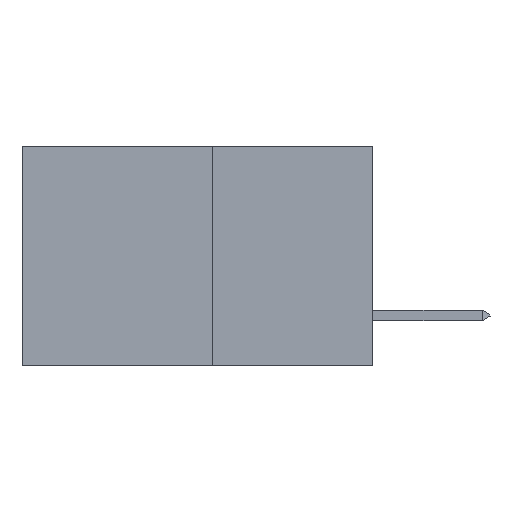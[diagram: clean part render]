
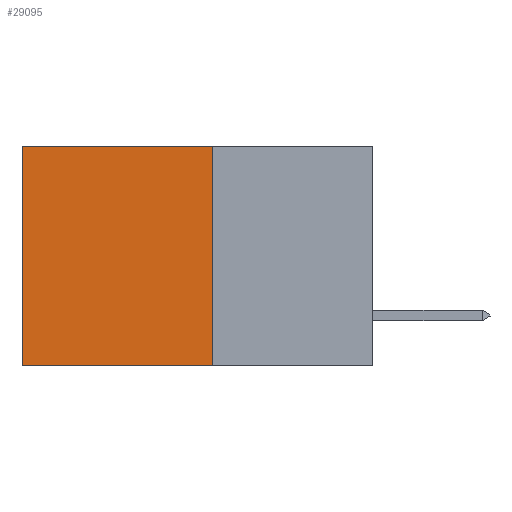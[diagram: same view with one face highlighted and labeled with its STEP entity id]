
A CAD part, left-side view. The second image highlights one B-rep face of the part: STEP entity #29095.
In plain terms, the highlighted planar face has unit normal (-1, 0, 0).
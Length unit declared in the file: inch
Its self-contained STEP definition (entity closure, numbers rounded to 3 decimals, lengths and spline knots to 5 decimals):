
#721 = ORIENTED_EDGE ( 'NONE', *, *, #19564, .F. ) ;
#1201 = VECTOR ( 'NONE', #18726, 39.37008 ) ;
#2480 = DIRECTION ( 'NONE',  ( 0., 0., -1. ) ) ;
#2927 = LINE ( 'NONE', #10168, #8708 ) ;
#3611 = VERTEX_POINT ( 'NONE', #15338 ) ;
#4893 = CARTESIAN_POINT ( 'NONE',  ( 0.277, 0.59, 0. ) ) ;
#6789 = EDGE_CURVE ( 'NONE', #23479, #3611, #12079, .T. ) ;
#7632 = CARTESIAN_POINT ( 'NONE',  ( 0.277, 0.27, -0.37 ) ) ;
#7766 = LINE ( 'NONE', #23638, #1201 ) ;
#7844 = CARTESIAN_POINT ( 'NONE',  ( 0.277, 0.59, -0.37 ) ) ;
#7878 = ORIENTED_EDGE ( 'NONE', *, *, #25058, .T. ) ;
#8621 = CARTESIAN_POINT ( 'NONE',  ( 0.277, 0.27, -0.37 ) ) ;
#8708 = VECTOR ( 'NONE', #20079, 39.37008 ) ;
#9586 = VECTOR ( 'NONE', #2480, 39.37008 ) ;
#10168 = CARTESIAN_POINT ( 'NONE',  ( 0.277, 0.27, -0.37 ) ) ;
#11098 = ORIENTED_EDGE ( 'NONE', *, *, #6789, .F. ) ;
#12079 = LINE ( 'NONE', #8621, #17922 ) ;
#12637 = DIRECTION ( 'NONE',  ( 1., 0., 0. ) ) ;
#13516 = DIRECTION ( 'NONE',  ( 0., 1., 0. ) ) ;
#15338 = CARTESIAN_POINT ( 'NONE',  ( 0.277, 0.59, -0.37 ) ) ;
#17259 = EDGE_LOOP ( 'NONE', ( #18206, #11098, #721, #7878 ) ) ;
#17922 = VECTOR ( 'NONE', #13516, 39.37008 ) ;
#18206 = ORIENTED_EDGE ( 'NONE', *, *, #26479, .T. ) ;
#18726 = DIRECTION ( 'NONE',  ( 0., 1., 0. ) ) ;
#19495 = VERTEX_POINT ( 'NONE', #4893 ) ;
#19564 = EDGE_CURVE ( 'NONE', #30369, #23479, #2927, .T. ) ;
#20079 = DIRECTION ( 'NONE',  ( 0., 0., -1. ) ) ;
#20743 = FACE_OUTER_BOUND ( 'NONE', #17259, .T. ) ;
#20803 = AXIS2_PLACEMENT_3D ( 'NONE', #7632, #12637, #29971 ) ;
#22065 = CARTESIAN_POINT ( 'NONE',  ( 0.277, 0.27, -0.37 ) ) ;
#23479 = VERTEX_POINT ( 'NONE', #22065 ) ;
#23638 = CARTESIAN_POINT ( 'NONE',  ( 0.277, 0.27, 0. ) ) ;
#25058 = EDGE_CURVE ( 'NONE', #30369, #19495, #7766, .T. ) ;
#26424 = CARTESIAN_POINT ( 'NONE',  ( 0.277, 0.27, 0. ) ) ;
#26479 = EDGE_CURVE ( 'NONE', #19495, #3611, #29401, .T. ) ;
#27534 = PLANE ( 'NONE',  #20803 ) ;
#29095 = ADVANCED_FACE ( 'NONE', ( #20743 ), #27534, .F. ) ;
#29401 = LINE ( 'NONE', #7844, #9586 ) ;
#29971 = DIRECTION ( 'NONE',  ( 0., 0., -1. ) ) ;
#30369 = VERTEX_POINT ( 'NONE', #26424 ) ;
